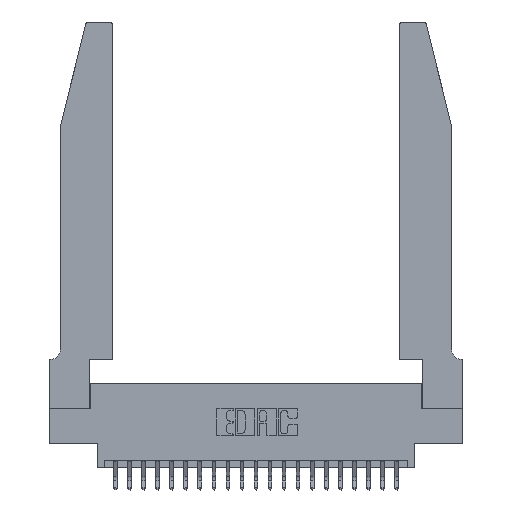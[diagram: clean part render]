
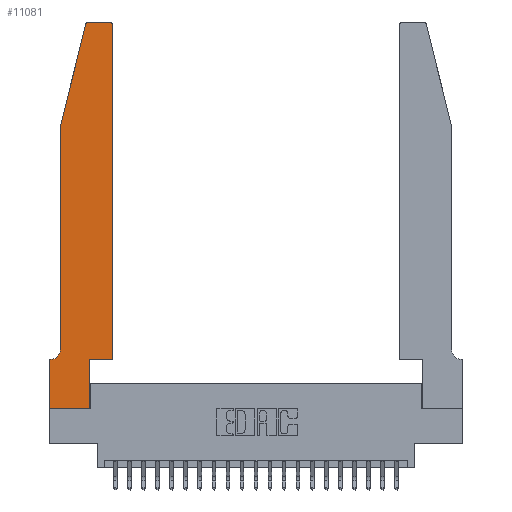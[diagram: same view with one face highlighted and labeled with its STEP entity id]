
A CAD part, top view. The second image highlights one B-rep face of the part: STEP entity #11081.
In plain terms, the highlighted planar face has unit normal (0, 0, 1).
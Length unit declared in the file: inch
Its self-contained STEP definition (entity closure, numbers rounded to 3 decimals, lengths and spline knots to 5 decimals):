
#236 = VERTEX_POINT ( 'NONE', #22347 ) ;
#246 = VERTEX_POINT ( 'NONE', #20194 ) ;
#374 = EDGE_CURVE ( 'NONE', #236, #3269, #19409, .T. ) ;
#840 = AXIS2_PLACEMENT_3D ( 'NONE', #11068, #23967, #12925 ) ;
#901 = CARTESIAN_POINT ( 'NONE',  ( 0.4505, 2.72, 0.37 ) ) ;
#1217 = VECTOR ( 'NONE', #18364, 39.37008 ) ;
#1615 = DIRECTION ( 'NONE',  ( 1., 0., 0. ) ) ;
#2257 = ORIENTED_EDGE ( 'NONE', *, *, #4213, .T. ) ;
#2300 = VERTEX_POINT ( 'NONE', #19071 ) ;
#2684 = CARTESIAN_POINT ( 'NONE',  ( 0.2605, 2.75, 0.37 ) ) ;
#2926 = CARTESIAN_POINT ( 'NONE',  ( 0.0055, 0.42, 0.37 ) ) ;
#3269 = VERTEX_POINT ( 'NONE', #4028 ) ;
#3611 = LINE ( 'NONE', #2684, #12558 ) ;
#3752 = CARTESIAN_POINT ( 'NONE',  ( 0.4505, 0.35, 0.37 ) ) ;
#3864 = LINE ( 'NONE', #3752, #8407 ) ;
#3891 = CARTESIAN_POINT ( 'NONE',  ( 0., 0., 0.37 ) ) ;
#4028 = CARTESIAN_POINT ( 'NONE',  ( 0.4505, 0.35, 0.37 ) ) ;
#4142 = VERTEX_POINT ( 'NONE', #7376 ) ;
#4213 = EDGE_CURVE ( 'NONE', #4142, #7940, #6961, .T. ) ;
#4300 = CARTESIAN_POINT ( 'NONE',  ( 0.284, 2.72, 0.37 ) ) ;
#4842 = DIRECTION ( 'NONE',  ( -1., 0., 0. ) ) ;
#4883 = EDGE_CURVE ( 'NONE', #19611, #6828, #6009, .T. ) ;
#5027 = EDGE_CURVE ( 'NONE', #18203, #12417, #3611, .T. ) ;
#5074 = CIRCLE ( 'NONE', #840, 0.03 ) ;
#5082 = LINE ( 'NONE', #22239, #14632 ) ;
#5118 = VECTOR ( 'NONE', #22437, 39.37008 ) ;
#5170 = PLANE ( 'NONE',  #12203 ) ;
#5808 = DIRECTION ( 'NONE',  ( 1., 0., 0. ) ) ;
#5921 = CARTESIAN_POINT ( 'NONE',  ( 0.0755, 2., 0.37 ) ) ;
#6009 = LINE ( 'NONE', #10027, #20977 ) ;
#6072 = VERTEX_POINT ( 'NONE', #22994 ) ;
#6246 = DIRECTION ( 'NONE',  ( 1., 0., 0. ) ) ;
#6739 = CARTESIAN_POINT ( 'NONE',  ( 0., 0.35, 0.37 ) ) ;
#6828 = VERTEX_POINT ( 'NONE', #19681 ) ;
#6961 = LINE ( 'NONE', #13245, #5118 ) ;
#7155 = DIRECTION ( 'NONE',  ( 0., 0., 1. ) ) ;
#7376 = CARTESIAN_POINT ( 'NONE',  ( 0.25487, 2.72718, 0.37 ) ) ;
#7404 = VECTOR ( 'NONE', #16485, 39.37008 ) ;
#7415 = EDGE_LOOP ( 'NONE', ( #24146, #20126, #2257, #12141, #12323, #15783, #10822, #18542, #11802, #22773, #19764, #14278 ) ) ;
#7784 = CARTESIAN_POINT ( 'NONE',  ( 0.284, 2.75, 0.37 ) ) ;
#7940 = VERTEX_POINT ( 'NONE', #5921 ) ;
#8407 = VECTOR ( 'NONE', #18829, 39.37008 ) ;
#8449 = EDGE_CURVE ( 'NONE', #6828, #6072, #21809, .T. ) ;
#10027 = CARTESIAN_POINT ( 'NONE',  ( 0., 0., 0.37 ) ) ;
#10329 = EDGE_CURVE ( 'NONE', #6072, #236, #13601, .T. ) ;
#10786 = VECTOR ( 'NONE', #5808, 39.37008 ) ;
#10822 = ORIENTED_EDGE ( 'NONE', *, *, #4883, .T. ) ;
#11068 = CARTESIAN_POINT ( 'NONE',  ( 0.4205, 2.72, 0.37 ) ) ;
#11081 = ADVANCED_FACE ( 'NONE', ( #21963 ), #5170, .T. ) ;
#11248 = CARTESIAN_POINT ( 'NONE',  ( 0.4505, 0.35, 0.37 ) ) ;
#11802 = ORIENTED_EDGE ( 'NONE', *, *, #10329, .T. ) ;
#12141 = ORIENTED_EDGE ( 'NONE', *, *, #15907, .T. ) ;
#12203 = AXIS2_PLACEMENT_3D ( 'NONE', #18370, #7155, #20210 ) ;
#12323 = ORIENTED_EDGE ( 'NONE', *, *, #17683, .T. ) ;
#12417 = VERTEX_POINT ( 'NONE', #7784 ) ;
#12509 = EDGE_CURVE ( 'NONE', #12417, #4142, #15435, .T. ) ;
#12558 = VECTOR ( 'NONE', #17851, 39.37008 ) ;
#12925 = DIRECTION ( 'NONE',  ( 1., 0., 0. ) ) ;
#13245 = CARTESIAN_POINT ( 'NONE',  ( 0.0755, 2., 0.37 ) ) ;
#13339 = CARTESIAN_POINT ( 'NONE',  ( 0.4205, 2.75, 0.37 ) ) ;
#13601 = LINE ( 'NONE', #23768, #7404 ) ;
#13727 = CIRCLE ( 'NONE', #17898, 0.07 ) ;
#13783 = DIRECTION ( 'NONE',  ( 0., -1., 0. ) ) ;
#14113 = AXIS2_PLACEMENT_3D ( 'NONE', #4300, #17538, #6246 ) ;
#14278 = ORIENTED_EDGE ( 'NONE', *, *, #17862, .T. ) ;
#14510 = VECTOR ( 'NONE', #1615, 39.37008 ) ;
#14632 = VECTOR ( 'NONE', #24070, 39.37008 ) ;
#15435 = CIRCLE ( 'NONE', #14113, 0.03 ) ;
#15783 = ORIENTED_EDGE ( 'NONE', *, *, #23041, .T. ) ;
#15907 = EDGE_CURVE ( 'NONE', #7940, #2300, #16459, .T. ) ;
#16208 = DIRECTION ( 'NONE',  ( 0., 0., -1. ) ) ;
#16429 = VERTEX_POINT ( 'NONE', #901 ) ;
#16459 = LINE ( 'NONE', #16529, #1217 ) ;
#16485 = DIRECTION ( 'NONE',  ( 0., 1., 0. ) ) ;
#16529 = CARTESIAN_POINT ( 'NONE',  ( 0.0755, 2., 0.37 ) ) ;
#17538 = DIRECTION ( 'NONE',  ( 0., 0., 1. ) ) ;
#17683 = EDGE_CURVE ( 'NONE', #2300, #246, #13727, .T. ) ;
#17851 = DIRECTION ( 'NONE',  ( -1., 0., 0. ) ) ;
#17862 = EDGE_CURVE ( 'NONE', #16429, #18203, #5074, .T. ) ;
#17898 = AXIS2_PLACEMENT_3D ( 'NONE', #2926, #16208, #4842 ) ;
#18203 = VERTEX_POINT ( 'NONE', #13339 ) ;
#18364 = DIRECTION ( 'NONE',  ( 0., -1., 0. ) ) ;
#18370 = CARTESIAN_POINT ( 'NONE',  ( 0., 0.35, 0.37 ) ) ;
#18542 = ORIENTED_EDGE ( 'NONE', *, *, #8449, .T. ) ;
#18829 = DIRECTION ( 'NONE',  ( 0., 1., 0. ) ) ;
#19071 = CARTESIAN_POINT ( 'NONE',  ( 0.0755, 0.42, 0.37 ) ) ;
#19409 = LINE ( 'NONE', #11248, #14510 ) ;
#19611 = VERTEX_POINT ( 'NONE', #6739 ) ;
#19681 = CARTESIAN_POINT ( 'NONE',  ( 0., 0., 0.37 ) ) ;
#19764 = ORIENTED_EDGE ( 'NONE', *, *, #24052, .T. ) ;
#20126 = ORIENTED_EDGE ( 'NONE', *, *, #12509, .T. ) ;
#20194 = CARTESIAN_POINT ( 'NONE',  ( 0.0055, 0.35, 0.37 ) ) ;
#20210 = DIRECTION ( 'NONE',  ( 1., 0., 0. ) ) ;
#20977 = VECTOR ( 'NONE', #13783, 39.37008 ) ;
#21809 = LINE ( 'NONE', #3891, #10786 ) ;
#21963 = FACE_OUTER_BOUND ( 'NONE', #7415, .T. ) ;
#22239 = CARTESIAN_POINT ( 'NONE',  ( 0.0755, 0.35, 0.37 ) ) ;
#22347 = CARTESIAN_POINT ( 'NONE',  ( 0.2865, 0.35, 0.37 ) ) ;
#22437 = DIRECTION ( 'NONE',  ( -0.239, -0.971, 0. ) ) ;
#22773 = ORIENTED_EDGE ( 'NONE', *, *, #374, .T. ) ;
#22994 = CARTESIAN_POINT ( 'NONE',  ( 0.2865, 0., 0.37 ) ) ;
#23041 = EDGE_CURVE ( 'NONE', #246, #19611, #5082, .T. ) ;
#23768 = CARTESIAN_POINT ( 'NONE',  ( 0.2865, 0.35, 0.37 ) ) ;
#23967 = DIRECTION ( 'NONE',  ( 0., 0., 1. ) ) ;
#24052 = EDGE_CURVE ( 'NONE', #3269, #16429, #3864, .T. ) ;
#24070 = DIRECTION ( 'NONE',  ( -1., 0., 0. ) ) ;
#24146 = ORIENTED_EDGE ( 'NONE', *, *, #5027, .T. ) ;
